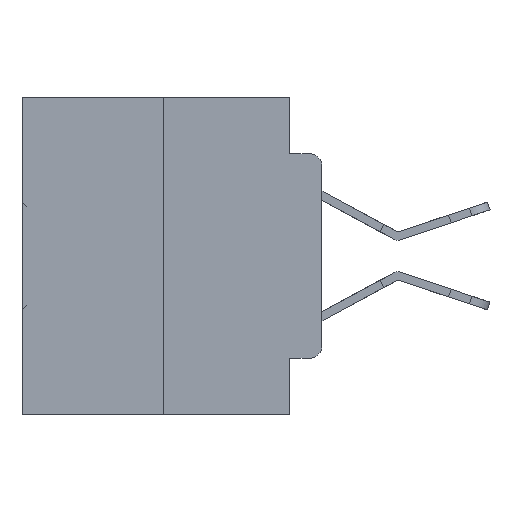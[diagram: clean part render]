
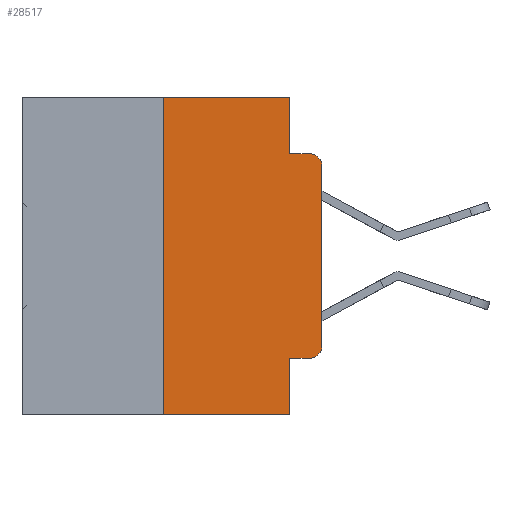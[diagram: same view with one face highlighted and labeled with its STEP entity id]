
A CAD part, left-side view. The second image highlights one B-rep face of the part: STEP entity #28517.
In plain terms, the highlighted planar face has unit normal (-1, 0, 0).
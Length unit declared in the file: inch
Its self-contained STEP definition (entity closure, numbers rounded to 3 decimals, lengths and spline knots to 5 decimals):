
#82 = VERTEX_POINT ( 'NONE', #20936 ) ;
#168 = CARTESIAN_POINT ( 'NONE',  ( 0., 0.473, 0. ) ) ;
#2381 = DIRECTION ( 'NONE',  ( -1., 0., 0. ) ) ;
#2791 = VERTEX_POINT ( 'NONE', #33077 ) ;
#3733 = ORIENTED_EDGE ( 'NONE', *, *, #28006, .T. ) ;
#4158 = CARTESIAN_POINT ( 'NONE',  ( 0., 0.051, -0.4115 ) ) ;
#4173 = LINE ( 'NONE', #13736, #24569 ) ;
#4957 = VERTEX_POINT ( 'NONE', #17342 ) ;
#5133 = AXIS2_PLACEMENT_3D ( 'NONE', #27907, #2381, #16449 ) ;
#5422 = VECTOR ( 'NONE', #12094, 39.37008 ) ;
#5518 = ORIENTED_EDGE ( 'NONE', *, *, #10863, .T. ) ;
#6818 = EDGE_CURVE ( 'NONE', #16865, #19496, #26668, .T. ) ;
#6962 = VERTEX_POINT ( 'NONE', #4158 ) ;
#7148 = EDGE_CURVE ( 'NONE', #6962, #25369, #35558, .T. ) ;
#7188 = LINE ( 'NONE', #9596, #5422 ) ;
#7590 = VECTOR ( 'NONE', #32493, 39.37008 ) ;
#7804 = DIRECTION ( 'NONE',  ( 0., -1., 0. ) ) ;
#8124 = DIRECTION ( 'NONE',  ( -1., 0., 0. ) ) ;
#8151 = EDGE_LOOP ( 'NONE', ( #5518, #9455, #30816, #26799, #26012, #32606, #20356, #11987, #18891, #3733 ) ) ;
#8805 = CARTESIAN_POINT ( 'NONE',  ( 0., 0.051, -0.5 ) ) ;
#9455 = ORIENTED_EDGE ( 'NONE', *, *, #10927, .T. ) ;
#9583 = CARTESIAN_POINT ( 'NONE',  ( 0., 0.051, -0.0885 ) ) ;
#9596 = CARTESIAN_POINT ( 'NONE',  ( 0., 0.051, 0. ) ) ;
#9691 = VECTOR ( 'NONE', #32596, 39.37008 ) ;
#9693 = DIRECTION ( 'NONE',  ( 0., 0., -1. ) ) ;
#9777 = VECTOR ( 'NONE', #7804, 39.37008 ) ;
#10323 = PLANE ( 'NONE',  #23766 ) ;
#10576 = LINE ( 'NONE', #12447, #9691 ) ;
#10863 = EDGE_CURVE ( 'NONE', #4957, #2791, #4173, .T. ) ;
#10927 = EDGE_CURVE ( 'NONE', #2791, #24303, #23669, .T. ) ;
#11691 = EDGE_CURVE ( 'NONE', #6962, #15829, #7188, .T. ) ;
#11987 = ORIENTED_EDGE ( 'NONE', *, *, #11691, .F. ) ;
#12094 = DIRECTION ( 'NONE',  ( 0., 0., -1. ) ) ;
#12447 = CARTESIAN_POINT ( 'NONE',  ( 0., 0.473, -0.5 ) ) ;
#13142 = CARTESIAN_POINT ( 'NONE',  ( 0., 0.473, 0. ) ) ;
#13736 = CARTESIAN_POINT ( 'NONE',  ( 0., 0., 0. ) ) ;
#14032 = DIRECTION ( 'NONE',  ( 0., 0., -1. ) ) ;
#14196 = VECTOR ( 'NONE', #9693, 39.37008 ) ;
#14210 = LINE ( 'NONE', #15557, #7590 ) ;
#15557 = CARTESIAN_POINT ( 'NONE',  ( 0., 0.25, 0. ) ) ;
#15829 = VERTEX_POINT ( 'NONE', #8805 ) ;
#16113 = DIRECTION ( 'NONE',  ( 0., 0., -1. ) ) ;
#16449 = DIRECTION ( 'NONE',  ( 0., 0., -1. ) ) ;
#16759 = VECTOR ( 'NONE', #25370, 39.37008 ) ;
#16865 = VERTEX_POINT ( 'NONE', #33833 ) ;
#17066 = CARTESIAN_POINT ( 'NONE',  ( 0., 0.02, -0.4115 ) ) ;
#17342 = CARTESIAN_POINT ( 'NONE',  ( 0., 0., -0.3915 ) ) ;
#17513 = CARTESIAN_POINT ( 'NONE',  ( 0., 0.02, -0.0885 ) ) ;
#17563 = VECTOR ( 'NONE', #32202, 39.37008 ) ;
#17640 = LINE ( 'NONE', #168, #16759 ) ;
#18891 = ORIENTED_EDGE ( 'NONE', *, *, #7148, .T. ) ;
#19496 = VERTEX_POINT ( 'NONE', #29310 ) ;
#20356 = ORIENTED_EDGE ( 'NONE', *, *, #32699, .T. ) ;
#20720 = CIRCLE ( 'NONE', #24712, 0.02 ) ;
#20936 = CARTESIAN_POINT ( 'NONE',  ( 0., 0.25, 0. ) ) ;
#22525 = DIRECTION ( 'NONE',  ( 0., 0., 1. ) ) ;
#23340 = CARTESIAN_POINT ( 'NONE',  ( 0., 0.051, 0. ) ) ;
#23344 = LINE ( 'NONE', #9583, #17563 ) ;
#23669 = CIRCLE ( 'NONE', #5133, 0.02 ) ;
#23766 = AXIS2_PLACEMENT_3D ( 'NONE', #13142, #24596, #16113 ) ;
#24303 = VERTEX_POINT ( 'NONE', #17513 ) ;
#24569 = VECTOR ( 'NONE', #22525, 39.37008 ) ;
#24596 = DIRECTION ( 'NONE',  ( 1., 0., 0. ) ) ;
#24712 = AXIS2_PLACEMENT_3D ( 'NONE', #25493, #8124, #14032 ) ;
#24928 = EDGE_CURVE ( 'NONE', #19496, #24303, #23344, .T. ) ;
#25070 = CARTESIAN_POINT ( 'NONE',  ( 0., 0.051, -0.4115 ) ) ;
#25369 = VERTEX_POINT ( 'NONE', #17066 ) ;
#25370 = DIRECTION ( 'NONE',  ( 0., -1., 0. ) ) ;
#25493 = CARTESIAN_POINT ( 'NONE',  ( 0., 0.02, -0.3915 ) ) ;
#26012 = ORIENTED_EDGE ( 'NONE', *, *, #30489, .F. ) ;
#26668 = LINE ( 'NONE', #23340, #14196 ) ;
#26799 = ORIENTED_EDGE ( 'NONE', *, *, #6818, .F. ) ;
#27237 = VERTEX_POINT ( 'NONE', #31545 ) ;
#27907 = CARTESIAN_POINT ( 'NONE',  ( 0., 0.02, -0.1085 ) ) ;
#28006 = EDGE_CURVE ( 'NONE', #25369, #4957, #20720, .T. ) ;
#28517 = ADVANCED_FACE ( 'NONE', ( #32095 ), #10323, .F. ) ;
#29310 = CARTESIAN_POINT ( 'NONE',  ( 0., 0.051, -0.0885 ) ) ;
#30489 = EDGE_CURVE ( 'NONE', #82, #16865, #17640, .T. ) ;
#30816 = ORIENTED_EDGE ( 'NONE', *, *, #24928, .F. ) ;
#31545 = CARTESIAN_POINT ( 'NONE',  ( 0., 0.25, -0.5 ) ) ;
#32095 = FACE_OUTER_BOUND ( 'NONE', #8151, .T. ) ;
#32202 = DIRECTION ( 'NONE',  ( 0., -1., 0. ) ) ;
#32493 = DIRECTION ( 'NONE',  ( 0., 0., 1. ) ) ;
#32596 = DIRECTION ( 'NONE',  ( 0., -1., 0. ) ) ;
#32606 = ORIENTED_EDGE ( 'NONE', *, *, #34353, .F. ) ;
#32699 = EDGE_CURVE ( 'NONE', #27237, #15829, #10576, .T. ) ;
#33077 = CARTESIAN_POINT ( 'NONE',  ( 0., 0., -0.1085 ) ) ;
#33833 = CARTESIAN_POINT ( 'NONE',  ( 0., 0.051, 0. ) ) ;
#34353 = EDGE_CURVE ( 'NONE', #27237, #82, #14210, .T. ) ;
#35558 = LINE ( 'NONE', #25070, #9777 ) ;
